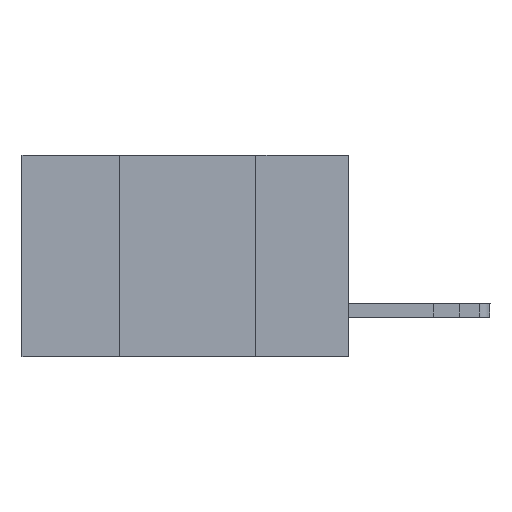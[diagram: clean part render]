
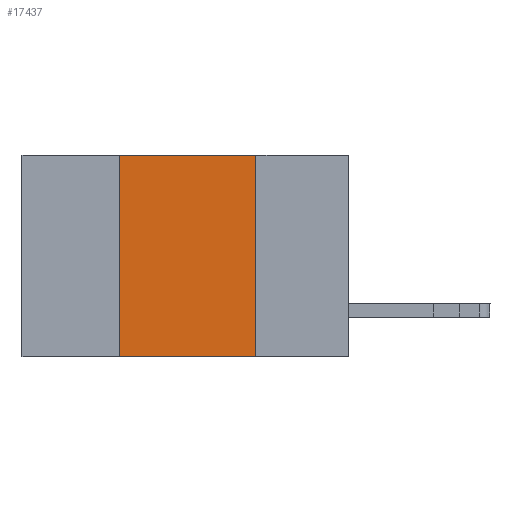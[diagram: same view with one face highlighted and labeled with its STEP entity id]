
A CAD part, left-side view. The second image highlights one B-rep face of the part: STEP entity #17437.
In plain terms, the highlighted planar face has unit normal (-1, 0, 0).
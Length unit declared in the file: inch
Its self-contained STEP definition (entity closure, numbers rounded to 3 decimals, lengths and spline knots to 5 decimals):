
#49 = EDGE_CURVE ( 'NONE', #5045, #434, #7444, .T. ) ;
#407 = CARTESIAN_POINT ( 'NONE',  ( 0., 0.17, 0. ) ) ;
#434 = VERTEX_POINT ( 'NONE', #6148 ) ;
#1271 = VERTEX_POINT ( 'NONE', #407 ) ;
#1425 = VERTEX_POINT ( 'NONE', #7495 ) ;
#1435 = CARTESIAN_POINT ( 'NONE',  ( 0., 0.6, -0.37 ) ) ;
#4311 = FACE_OUTER_BOUND ( 'NONE', #16922, .T. ) ;
#4412 = VECTOR ( 'NONE', #14347, 39.37008 ) ;
#5045 = VERTEX_POINT ( 'NONE', #17033 ) ;
#5098 = DIRECTION ( 'NONE',  ( 1., 0., 0. ) ) ;
#5242 = PLANE ( 'NONE',  #9271 ) ;
#6148 = CARTESIAN_POINT ( 'NONE',  ( 0., 0.42, 0. ) ) ;
#6556 = DIRECTION ( 'NONE',  ( 0., -1., 0. ) ) ;
#6608 = EDGE_CURVE ( 'NONE', #1271, #1425, #12172, .T. ) ;
#6982 = VECTOR ( 'NONE', #15895, 39.37008 ) ;
#7444 = LINE ( 'NONE', #10025, #6982 ) ;
#7495 = CARTESIAN_POINT ( 'NONE',  ( 0., 0.17, -0.37 ) ) ;
#7827 = ORIENTED_EDGE ( 'NONE', *, *, #6608, .F. ) ;
#8225 = DIRECTION ( 'NONE',  ( 0., 0., -1. ) ) ;
#8321 = CARTESIAN_POINT ( 'NONE',  ( 0., 0.17, 0. ) ) ;
#8774 = EDGE_CURVE ( 'NONE', #5045, #1425, #13476, .T. ) ;
#9271 = AXIS2_PLACEMENT_3D ( 'NONE', #9639, #5098, #8225 ) ;
#9639 = CARTESIAN_POINT ( 'NONE',  ( 0., 0.6, 0. ) ) ;
#10025 = CARTESIAN_POINT ( 'NONE',  ( 0., 0.42, 0. ) ) ;
#10254 = DIRECTION ( 'NONE',  ( 0., -1., 0. ) ) ;
#12172 = LINE ( 'NONE', #8321, #4412 ) ;
#13476 = LINE ( 'NONE', #1435, #16415 ) ;
#13745 = ORIENTED_EDGE ( 'NONE', *, *, #49, .F. ) ;
#14135 = LINE ( 'NONE', #18625, #18431 ) ;
#14347 = DIRECTION ( 'NONE',  ( 0., 0., -1. ) ) ;
#14528 = ORIENTED_EDGE ( 'NONE', *, *, #8774, .T. ) ;
#15489 = ORIENTED_EDGE ( 'NONE', *, *, #18105, .F. ) ;
#15895 = DIRECTION ( 'NONE',  ( 0., 0., 1. ) ) ;
#16415 = VECTOR ( 'NONE', #10254, 39.37008 ) ;
#16922 = EDGE_LOOP ( 'NONE', ( #7827, #15489, #13745, #14528 ) ) ;
#17033 = CARTESIAN_POINT ( 'NONE',  ( 0., 0.42, -0.37 ) ) ;
#17437 = ADVANCED_FACE ( 'NONE', ( #4311 ), #5242, .F. ) ;
#18105 = EDGE_CURVE ( 'NONE', #434, #1271, #14135, .T. ) ;
#18431 = VECTOR ( 'NONE', #6556, 39.37008 ) ;
#18625 = CARTESIAN_POINT ( 'NONE',  ( 0., 0.6, 0. ) ) ;
